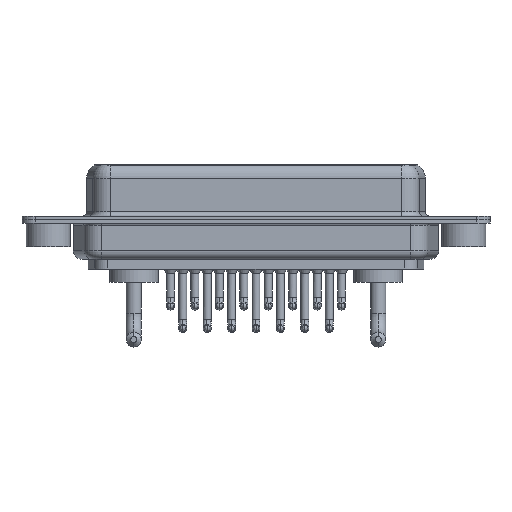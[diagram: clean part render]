
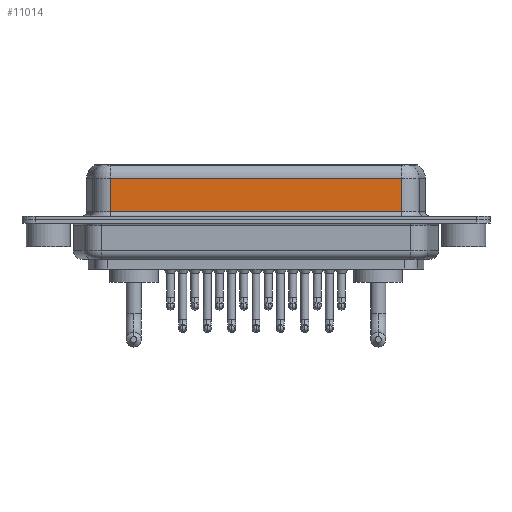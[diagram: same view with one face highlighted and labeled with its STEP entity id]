
A CAD part, front view. The second image highlights one B-rep face of the part: STEP entity #11014.
In plain terms, the highlighted planar face has unit normal (0, -1, 0).
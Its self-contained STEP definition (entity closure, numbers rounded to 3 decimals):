
#795 = ORIENTED_EDGE ( 'NONE', *, *, #3514, .T. ) ;
#1066 = FACE_OUTER_BOUND ( 'NONE', #5900, .T. ) ;
#1169 = AXIS2_PLACEMENT_3D ( 'NONE', #18917, #17040, #20289 ) ;
#1422 = CARTESIAN_POINT ( 'NONE',  ( 7.013, -3.95, 0.9 ) ) ;
#1431 = ORIENTED_EDGE ( 'NONE', *, *, #19931, .F. ) ;
#2007 = ORIENTED_EDGE ( 'NONE', *, *, #16116, .T. ) ;
#2219 = VERTEX_POINT ( 'NONE', #1422 ) ;
#3514 = EDGE_CURVE ( 'NONE', #7079, #2219, #11283, .T. ) ;
#4724 = VERTEX_POINT ( 'NONE', #7047 ) ;
#5900 = EDGE_LOOP ( 'NONE', ( #1431, #7415, #795, #2007 ) ) ;
#6709 = EDGE_CURVE ( 'NONE', #4724, #7079, #9252, .T. ) ;
#7047 = CARTESIAN_POINT ( 'NONE',  ( 40.037, -3.95, 4.65 ) ) ;
#7079 = VERTEX_POINT ( 'NONE', #10497 ) ;
#7232 = DIRECTION ( 'NONE',  ( 1., 0., 0. ) ) ;
#7415 = ORIENTED_EDGE ( 'NONE', *, *, #6709, .T. ) ;
#8838 = CARTESIAN_POINT ( 'NONE',  ( 40.037, -3.95, 0.9 ) ) ;
#9046 = DIRECTION ( 'NONE',  ( -1., 0., 0. ) ) ;
#9252 = LINE ( 'NONE', #20325, #14889 ) ;
#10497 = CARTESIAN_POINT ( 'NONE',  ( 7.013, -3.95, 4.65 ) ) ;
#10585 = PLANE ( 'NONE',  #1169 ) ;
#11014 = ADVANCED_FACE ( 'NONE', ( #1066 ), #10585, .F. ) ;
#11283 = LINE ( 'NONE', #20657, #11481 ) ;
#11481 = VECTOR ( 'NONE', #12884, 1000. ) ;
#12327 = LINE ( 'NONE', #8838, #19908 ) ;
#12884 = DIRECTION ( 'NONE',  ( 0., 0., -1. ) ) ;
#14273 = DIRECTION ( 'NONE',  ( 0., 0., -1. ) ) ;
#14889 = VECTOR ( 'NONE', #9046, 1000. ) ;
#15741 = VECTOR ( 'NONE', #14273, 1000. ) ;
#16116 = EDGE_CURVE ( 'NONE', #2219, #17953, #12327, .T. ) ;
#17040 = DIRECTION ( 'NONE',  ( 0., 1., 0. ) ) ;
#17724 = CARTESIAN_POINT ( 'NONE',  ( 40.037, -3.95, 6.4 ) ) ;
#17953 = VERTEX_POINT ( 'NONE', #18227 ) ;
#18227 = CARTESIAN_POINT ( 'NONE',  ( 40.037, -3.95, 0.9 ) ) ;
#18917 = CARTESIAN_POINT ( 'NONE',  ( 40.037, -3.95, 6.4 ) ) ;
#19908 = VECTOR ( 'NONE', #7232, 1000. ) ;
#19931 = EDGE_CURVE ( 'NONE', #4724, #17953, #20892, .T. ) ;
#20289 = DIRECTION ( 'NONE',  ( 0., 0., 1. ) ) ;
#20325 = CARTESIAN_POINT ( 'NONE',  ( 40.037, -3.95, 4.65 ) ) ;
#20657 = CARTESIAN_POINT ( 'NONE',  ( 7.013, -3.95, 6.4 ) ) ;
#20892 = LINE ( 'NONE', #17724, #15741 ) ;
